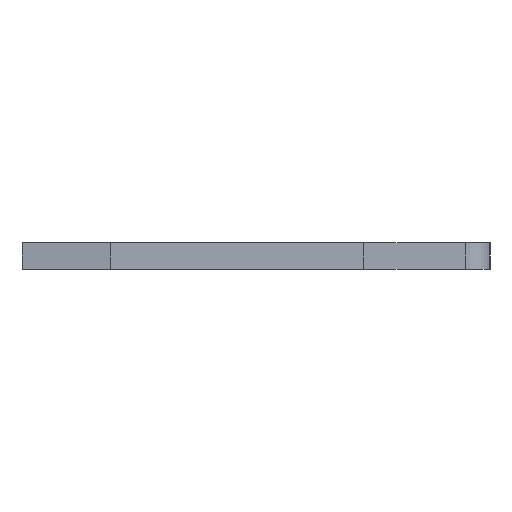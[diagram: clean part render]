
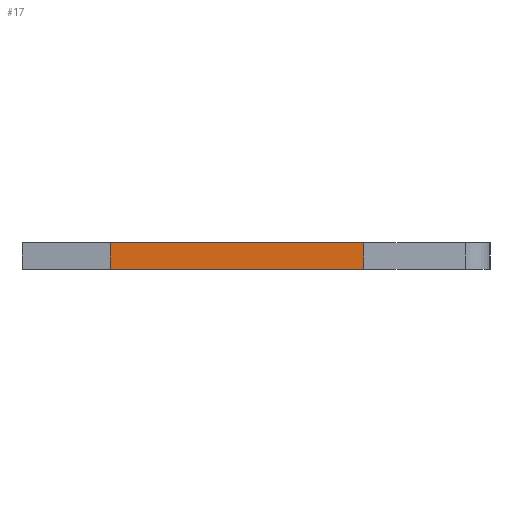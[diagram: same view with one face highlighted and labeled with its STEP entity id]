
A CAD part, left-side view. The second image highlights one B-rep face of the part: STEP entity #17.
In plain terms, the highlighted face is planar.
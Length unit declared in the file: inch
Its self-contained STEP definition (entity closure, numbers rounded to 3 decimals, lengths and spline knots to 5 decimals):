
#17 = ADVANCED_FACE ( 'NONE', ( #670 ), #1395, .F. ) ;
#55 = ORIENTED_EDGE ( 'NONE', *, *, #1966, .F. ) ;
#76 = EDGE_LOOP ( 'NONE', ( #2051, #995, #55, #196 ) ) ;
#155 = VERTEX_POINT ( 'NONE', #575 ) ;
#196 = ORIENTED_EDGE ( 'NONE', *, *, #729, .T. ) ;
#276 = LINE ( 'NONE', #655, #554 ) ;
#290 = CARTESIAN_POINT ( 'NONE',  ( -0.013, -0.099, -0.0575 ) ) ;
#377 = CARTESIAN_POINT ( 'NONE',  ( -0.013, 0.146, -0.0575 ) ) ;
#554 = VECTOR ( 'NONE', #1802, 39.37008 ) ;
#575 = CARTESIAN_POINT ( 'NONE',  ( 0.013, -0.099, -0.0575 ) ) ;
#655 = CARTESIAN_POINT ( 'NONE',  ( 0.013, 0.146, -0.0575 ) ) ;
#664 = LINE ( 'NONE', #377, #687 ) ;
#670 = FACE_OUTER_BOUND ( 'NONE', #76, .T. ) ;
#687 = VECTOR ( 'NONE', #1852, 39.37008 ) ;
#729 = EDGE_CURVE ( 'NONE', #155, #1822, #1015, .T. ) ;
#819 = DIRECTION ( 'NONE',  ( -1., 0., 0. ) ) ;
#834 = VECTOR ( 'NONE', #819, 39.37008 ) ;
#868 = CARTESIAN_POINT ( 'NONE',  ( 0.013, 0.146, -0.0575 ) ) ;
#892 = EDGE_CURVE ( 'NONE', #1822, #1608, #664, .T. ) ;
#995 = ORIENTED_EDGE ( 'NONE', *, *, #1976, .F. ) ;
#1015 = LINE ( 'NONE', #1979, #1765 ) ;
#1194 = LINE ( 'NONE', #1638, #834 ) ;
#1302 = CARTESIAN_POINT ( 'NONE',  ( -0.013, 0.146, -0.0575 ) ) ;
#1395 = PLANE ( 'NONE',  #1444 ) ;
#1444 = AXIS2_PLACEMENT_3D ( 'NONE', #868, #1884, #1532 ) ;
#1464 = VERTEX_POINT ( 'NONE', #1551 ) ;
#1491 = DIRECTION ( 'NONE',  ( -1., 0., 0. ) ) ;
#1532 = DIRECTION ( 'NONE',  ( 1., 0., 0. ) ) ;
#1551 = CARTESIAN_POINT ( 'NONE',  ( 0.013, 0.146, -0.0575 ) ) ;
#1608 = VERTEX_POINT ( 'NONE', #1302 ) ;
#1638 = CARTESIAN_POINT ( 'NONE',  ( 0.013, 0.146, -0.0575 ) ) ;
#1765 = VECTOR ( 'NONE', #1491, 39.37008 ) ;
#1802 = DIRECTION ( 'NONE',  ( 0., 1., 0. ) ) ;
#1822 = VERTEX_POINT ( 'NONE', #290 ) ;
#1852 = DIRECTION ( 'NONE',  ( 0., 1., 0. ) ) ;
#1884 = DIRECTION ( 'NONE',  ( 0., 0., 1. ) ) ;
#1966 = EDGE_CURVE ( 'NONE', #155, #1464, #276, .T. ) ;
#1976 = EDGE_CURVE ( 'NONE', #1464, #1608, #1194, .T. ) ;
#1979 = CARTESIAN_POINT ( 'NONE',  ( 0.013, -0.099, -0.0575 ) ) ;
#2051 = ORIENTED_EDGE ( 'NONE', *, *, #892, .T. ) ;
